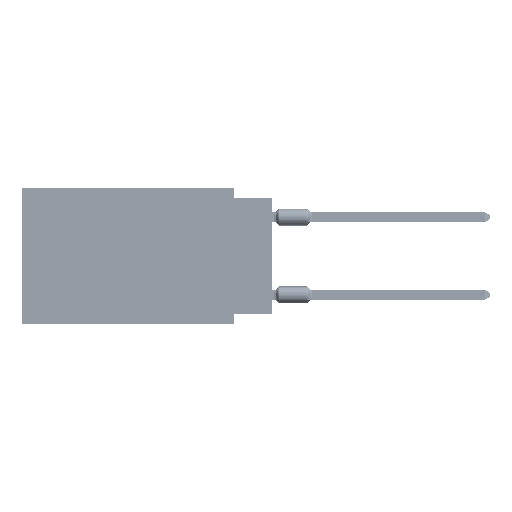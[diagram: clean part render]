
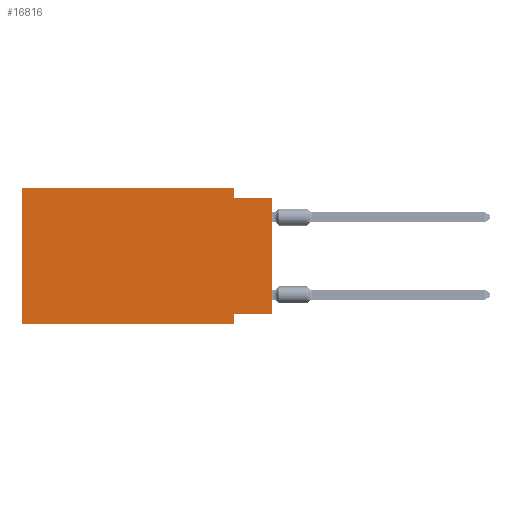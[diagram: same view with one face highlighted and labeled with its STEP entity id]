
A CAD part, left-side view. The second image highlights one B-rep face of the part: STEP entity #16816.
In plain terms, the highlighted planar face has unit normal (-1, 0, 0).
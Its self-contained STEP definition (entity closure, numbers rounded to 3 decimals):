
#2654 = ORIENTED_EDGE ( 'NONE', *, *, #41083, .F. ) ;
#4512 = CARTESIAN_POINT ( 'NONE',  ( 0., 16.383, 0. ) ) ;
#7471 = EDGE_CURVE ( 'NONE', #75946, #95062, #8943, .T. ) ;
#7865 = DIRECTION ( 'NONE',  ( 0., 0., 1. ) ) ;
#8815 = DIRECTION ( 'NONE',  ( 0., -1., 0. ) ) ;
#8943 = LINE ( 'NONE', #66754, #34278 ) ;
#10920 = CARTESIAN_POINT ( 'NONE',  ( 0., 2.54, -8.89 ) ) ;
#11447 = CARTESIAN_POINT ( 'NONE',  ( 0., 2.54, -0.635 ) ) ;
#11847 = DIRECTION ( 'NONE',  ( 1., 0., 0. ) ) ;
#12510 = CARTESIAN_POINT ( 'NONE',  ( 0., 0., -0.635 ) ) ;
#13748 = EDGE_CURVE ( 'NONE', #62250, #95493, #36667, .T. ) ;
#16214 = ORIENTED_EDGE ( 'NONE', *, *, #37282, .F. ) ;
#16816 = ADVANCED_FACE ( 'NONE', ( #89102 ), #64553, .F. ) ;
#17730 = CARTESIAN_POINT ( 'NONE',  ( 0., 0., -8.255 ) ) ;
#21214 = VECTOR ( 'NONE', #81756, 1000. ) ;
#23073 = DIRECTION ( 'NONE',  ( 0., 0., -1. ) ) ;
#23555 = LINE ( 'NONE', #56840, #94976 ) ;
#26735 = DIRECTION ( 'NONE',  ( 0., 0., -1. ) ) ;
#31516 = CARTESIAN_POINT ( 'NONE',  ( 0., 2.54, -8.255 ) ) ;
#32579 = ORIENTED_EDGE ( 'NONE', *, *, #63177, .F. ) ;
#33263 = VECTOR ( 'NONE', #87067, 1000. ) ;
#34278 = VECTOR ( 'NONE', #7865, 1000. ) ;
#36544 = LINE ( 'NONE', #10920, #41200 ) ;
#36667 = LINE ( 'NONE', #87403, #56020 ) ;
#37282 = EDGE_CURVE ( 'NONE', #105087, #60678, #36544, .T. ) ;
#39449 = CARTESIAN_POINT ( 'NONE',  ( 0., 16.383, 0. ) ) ;
#41083 = EDGE_CURVE ( 'NONE', #95493, #104076, #53970, .T. ) ;
#41200 = VECTOR ( 'NONE', #26735, 1000. ) ;
#42060 = EDGE_CURVE ( 'NONE', #87852, #105087, #81338, .T. ) ;
#45054 = CARTESIAN_POINT ( 'NONE',  ( 0., 0., 0. ) ) ;
#48796 = DIRECTION ( 'NONE',  ( 0., -1., 0. ) ) ;
#49648 = VECTOR ( 'NONE', #48796, 1000. ) ;
#52849 = EDGE_CURVE ( 'NONE', #75946, #60678, #63171, .T. ) ;
#53970 = LINE ( 'NONE', #12510, #21214 ) ;
#55043 = CARTESIAN_POINT ( 'NONE',  ( 0., 16.383, -8.89 ) ) ;
#55526 = ORIENTED_EDGE ( 'NONE', *, *, #71973, .T. ) ;
#56020 = VECTOR ( 'NONE', #62845, 1000. ) ;
#56237 = AXIS2_PLACEMENT_3D ( 'NONE', #39449, #11847, #23073 ) ;
#56786 = CARTESIAN_POINT ( 'NONE',  ( 0., 0., -8.255 ) ) ;
#56840 = CARTESIAN_POINT ( 'NONE',  ( 0., 16.383, 0. ) ) ;
#60678 = VERTEX_POINT ( 'NONE', #83048 ) ;
#61418 = LINE ( 'NONE', #45054, #33263 ) ;
#61928 = ORIENTED_EDGE ( 'NONE', *, *, #7471, .F. ) ;
#62250 = VERTEX_POINT ( 'NONE', #73244 ) ;
#62330 = EDGE_LOOP ( 'NONE', ( #55526, #2654, #89555, #32579, #61928, #88522, #16214, #81557 ) ) ;
#62845 = DIRECTION ( 'NONE',  ( 0., 0., -1. ) ) ;
#63171 = LINE ( 'NONE', #73887, #49648 ) ;
#63177 = EDGE_CURVE ( 'NONE', #95062, #62250, #23555, .T. ) ;
#64553 = PLANE ( 'NONE',  #56237 ) ;
#66754 = CARTESIAN_POINT ( 'NONE',  ( 0., 16.383, 0. ) ) ;
#71973 = EDGE_CURVE ( 'NONE', #87852, #104076, #61418, .T. ) ;
#73159 = DIRECTION ( 'NONE',  ( 0., 1., 0. ) ) ;
#73244 = CARTESIAN_POINT ( 'NONE',  ( 0., 2.54, 0. ) ) ;
#73887 = CARTESIAN_POINT ( 'NONE',  ( 0., 16.383, -8.89 ) ) ;
#75946 = VERTEX_POINT ( 'NONE', #55043 ) ;
#80474 = VECTOR ( 'NONE', #73159, 1000. ) ;
#81338 = LINE ( 'NONE', #56786, #80474 ) ;
#81557 = ORIENTED_EDGE ( 'NONE', *, *, #42060, .F. ) ;
#81756 = DIRECTION ( 'NONE',  ( 0., -1., 0. ) ) ;
#83048 = CARTESIAN_POINT ( 'NONE',  ( 0., 2.54, -8.89 ) ) ;
#87067 = DIRECTION ( 'NONE',  ( 0., 0., 1. ) ) ;
#87403 = CARTESIAN_POINT ( 'NONE',  ( 0., 2.54, 0. ) ) ;
#87852 = VERTEX_POINT ( 'NONE', #17730 ) ;
#88522 = ORIENTED_EDGE ( 'NONE', *, *, #52849, .T. ) ;
#89102 = FACE_OUTER_BOUND ( 'NONE', #62330, .T. ) ;
#89555 = ORIENTED_EDGE ( 'NONE', *, *, #13748, .F. ) ;
#94976 = VECTOR ( 'NONE', #8815, 1000. ) ;
#95062 = VERTEX_POINT ( 'NONE', #4512 ) ;
#95493 = VERTEX_POINT ( 'NONE', #11447 ) ;
#100744 = CARTESIAN_POINT ( 'NONE',  ( 0., 0., -0.635 ) ) ;
#104076 = VERTEX_POINT ( 'NONE', #100744 ) ;
#105087 = VERTEX_POINT ( 'NONE', #31516 ) ;
